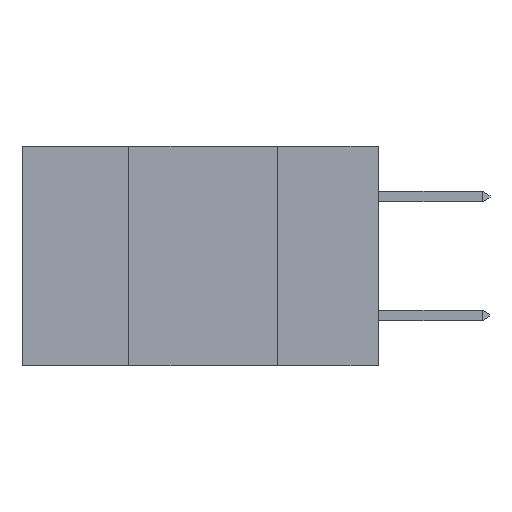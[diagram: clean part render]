
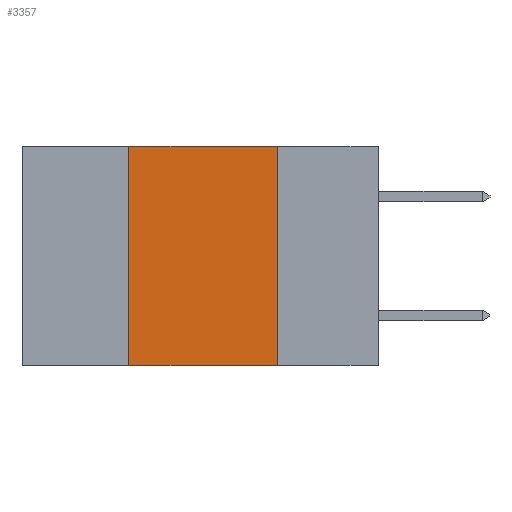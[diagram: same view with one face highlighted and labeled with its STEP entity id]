
A CAD part, left-side view. The second image highlights one B-rep face of the part: STEP entity #3357.
In plain terms, the highlighted planar face has unit normal (-1, 0, 0).
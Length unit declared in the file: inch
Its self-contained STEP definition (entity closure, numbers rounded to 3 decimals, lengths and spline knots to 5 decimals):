
#313 = FACE_OUTER_BOUND ( 'NONE', #7466, .T. ) ;
#975 = DIRECTION ( 'NONE',  ( 0., 0., -1. ) ) ;
#1083 = VECTOR ( 'NONE', #11036, 39.37008 ) ;
#1671 = LINE ( 'NONE', #14015, #7829 ) ;
#1942 = ORIENTED_EDGE ( 'NONE', *, *, #11850, .F. ) ;
#2345 = CARTESIAN_POINT ( 'NONE',  ( 0., 0.42, 0. ) ) ;
#3034 = CARTESIAN_POINT ( 'NONE',  ( 0., 0.17, 0. ) ) ;
#3153 = LINE ( 'NONE', #2345, #12082 ) ;
#3202 = VERTEX_POINT ( 'NONE', #10432 ) ;
#3357 = ADVANCED_FACE ( 'NONE', ( #313 ), #7084, .F. ) ;
#4610 = DIRECTION ( 'NONE',  ( 0., 0., -1. ) ) ;
#4876 = CARTESIAN_POINT ( 'NONE',  ( 0., 0.42, 0. ) ) ;
#6412 = VECTOR ( 'NONE', #975, 39.37008 ) ;
#7084 = PLANE ( 'NONE',  #14610 ) ;
#7466 = EDGE_LOOP ( 'NONE', ( #7696, #11277, #1942, #8465 ) ) ;
#7696 = ORIENTED_EDGE ( 'NONE', *, *, #11822, .F. ) ;
#7829 = VECTOR ( 'NONE', #10407, 39.37008 ) ;
#8465 = ORIENTED_EDGE ( 'NONE', *, *, #11921, .T. ) ;
#8531 = VERTEX_POINT ( 'NONE', #3034 ) ;
#8762 = CARTESIAN_POINT ( 'NONE',  ( 0., 0.42, -0.37 ) ) ;
#9705 = DIRECTION ( 'NONE',  ( 0., 0., 1. ) ) ;
#9708 = EDGE_CURVE ( 'NONE', #10092, #8531, #1671, .T. ) ;
#9858 = CARTESIAN_POINT ( 'NONE',  ( 0., 0.6, -0.37 ) ) ;
#10092 = VERTEX_POINT ( 'NONE', #4876 ) ;
#10407 = DIRECTION ( 'NONE',  ( 0., -1., 0. ) ) ;
#10432 = CARTESIAN_POINT ( 'NONE',  ( 0., 0.17, -0.37 ) ) ;
#10900 = LINE ( 'NONE', #9858, #1083 ) ;
#11036 = DIRECTION ( 'NONE',  ( 0., -1., 0. ) ) ;
#11277 = ORIENTED_EDGE ( 'NONE', *, *, #9708, .F. ) ;
#11311 = VERTEX_POINT ( 'NONE', #8762 ) ;
#11822 = EDGE_CURVE ( 'NONE', #8531, #3202, #12835, .T. ) ;
#11850 = EDGE_CURVE ( 'NONE', #11311, #10092, #3153, .T. ) ;
#11921 = EDGE_CURVE ( 'NONE', #11311, #3202, #10900, .T. ) ;
#12082 = VECTOR ( 'NONE', #9705, 39.37008 ) ;
#12835 = LINE ( 'NONE', #15562, #6412 ) ;
#14015 = CARTESIAN_POINT ( 'NONE',  ( 0., 0.6, 0. ) ) ;
#14610 = AXIS2_PLACEMENT_3D ( 'NONE', #15200, #15188, #4610 ) ;
#15188 = DIRECTION ( 'NONE',  ( 1., 0., 0. ) ) ;
#15200 = CARTESIAN_POINT ( 'NONE',  ( 0., 0.6, 0. ) ) ;
#15562 = CARTESIAN_POINT ( 'NONE',  ( 0., 0.17, 0. ) ) ;
